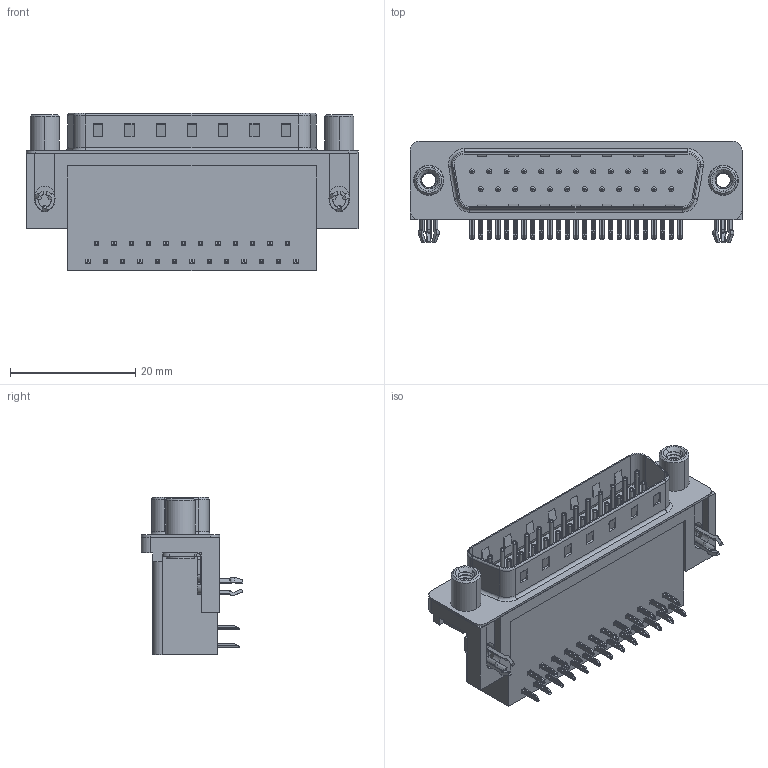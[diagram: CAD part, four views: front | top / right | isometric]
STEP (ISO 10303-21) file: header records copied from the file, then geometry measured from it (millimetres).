
FILE_DESCRIPTION (( 'STEP AP203' ), '1' );
FILE_NAME ('625-025-362-540.STEP', '2018-11-06T02:52:11', ( '' ), ( '' ), 'SwSTEP 2.0', 'SolidWorks 2016', '' );
FILE_SCHEMA (( 'CONFIG_CONTROL_DESIGN' ));
Length unit declared in the file: millimetre
Products named in the file (7): 625 Contact Top; 625 3 Prong Board Lock; 625 Round Threaded Standoff; 625-025-362-540; 625 Housing_25 Socket; 625 Shell_25 Socket; 625 Contact Bottom
Assembly tree (31 placements, depth 2):
  625-025-362-540
    625 Housing_25 Socket
    625 Shell_25 Socket
    625 Contact Bottom  x12
    625 Contact Top  x13
    625 3 Prong Board Lock  x2
    625 Round Threaded Standoff  x2
Bounding box: 53.04 x 16.25 x 25.16 mm (x, y, z)
Volume: 9263.3 mm3; surface area: 9121.7 mm2
Topology: 31 solids, 31 shells, 2363 faces, 5921 edges, 3675 vertices
Faces by surface type: plane 1435, cylinder 675, torus 189, cone 48, bspline 16
Entity records: 24577 total; most frequent: CARTESIAN_POINT 5659, DIRECTION 3694, ORIENTED_EDGE 3584, EDGE_CURVE 1792, AXIS2_PLACEMENT_3D 1234, LINE 1226, VECTOR 1226, VERTEX_POINT 1155
